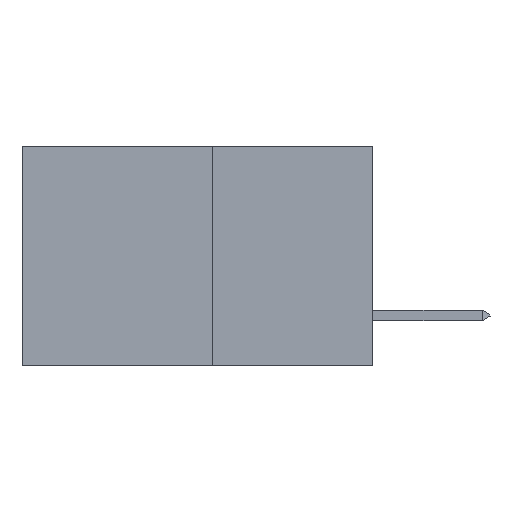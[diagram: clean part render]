
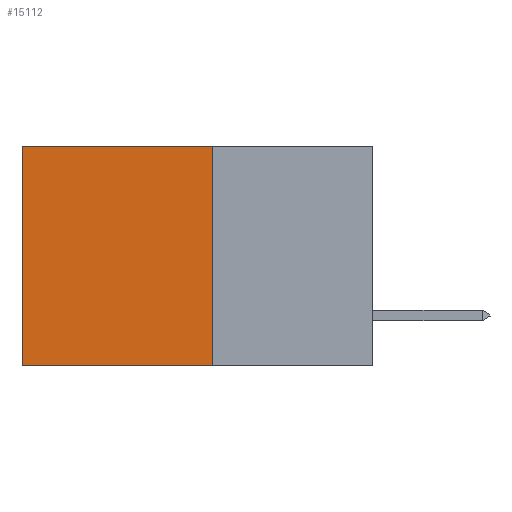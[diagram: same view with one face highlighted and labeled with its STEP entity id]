
A CAD part, left-side view. The second image highlights one B-rep face of the part: STEP entity #15112.
In plain terms, the highlighted planar face has unit normal (-1, 0, 0).
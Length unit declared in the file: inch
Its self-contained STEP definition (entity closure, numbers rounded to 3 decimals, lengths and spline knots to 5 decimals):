
#488 = EDGE_LOOP ( 'NONE', ( #20246, #15571, #25348, #21650 ) ) ;
#1628 = VERTEX_POINT ( 'NONE', #17150 ) ;
#3722 = VECTOR ( 'NONE', #17400, 39.37008 ) ;
#3807 = CARTESIAN_POINT ( 'NONE',  ( 0.277, 0.59, 0. ) ) ;
#5241 = FACE_OUTER_BOUND ( 'NONE', #488, .T. ) ;
#7103 = VERTEX_POINT ( 'NONE', #3807 ) ;
#7363 = VECTOR ( 'NONE', #7800, 39.37008 ) ;
#7687 = CARTESIAN_POINT ( 'NONE',  ( 0.277, 0.59, -0.37 ) ) ;
#7800 = DIRECTION ( 'NONE',  ( 0., 0., -1. ) ) ;
#8806 = DIRECTION ( 'NONE',  ( 0., 1., 0. ) ) ;
#8947 = CARTESIAN_POINT ( 'NONE',  ( 0.277, 0.27, 0. ) ) ;
#9897 = CARTESIAN_POINT ( 'NONE',  ( 0.277, 0.27, -0.37 ) ) ;
#10000 = CARTESIAN_POINT ( 'NONE',  ( 0.277, 0.27, -0.37 ) ) ;
#11214 = EDGE_CURVE ( 'NONE', #18471, #1628, #12854, .T. ) ;
#12854 = LINE ( 'NONE', #15002, #23775 ) ;
#13082 = LINE ( 'NONE', #9897, #7363 ) ;
#13847 = DIRECTION ( 'NONE',  ( 0., 0., -1. ) ) ;
#14249 = LINE ( 'NONE', #7687, #24519 ) ;
#14829 = CARTESIAN_POINT ( 'NONE',  ( 0.277, 0.27, 0. ) ) ;
#15002 = CARTESIAN_POINT ( 'NONE',  ( 0.277, 0.27, -0.37 ) ) ;
#15082 = LINE ( 'NONE', #8947, #3722 ) ;
#15112 = ADVANCED_FACE ( 'NONE', ( #5241 ), #22031, .F. ) ;
#15571 = ORIENTED_EDGE ( 'NONE', *, *, #11214, .F. ) ;
#16810 = AXIS2_PLACEMENT_3D ( 'NONE', #24074, #26175, #13847 ) ;
#17150 = CARTESIAN_POINT ( 'NONE',  ( 0.277, 0.59, -0.37 ) ) ;
#17400 = DIRECTION ( 'NONE',  ( 0., 1., 0. ) ) ;
#18288 = EDGE_CURVE ( 'NONE', #19373, #7103, #15082, .T. ) ;
#18471 = VERTEX_POINT ( 'NONE', #10000 ) ;
#19373 = VERTEX_POINT ( 'NONE', #14829 ) ;
#20246 = ORIENTED_EDGE ( 'NONE', *, *, #24473, .T. ) ;
#21650 = ORIENTED_EDGE ( 'NONE', *, *, #18288, .T. ) ;
#22031 = PLANE ( 'NONE',  #16810 ) ;
#22399 = EDGE_CURVE ( 'NONE', #19373, #18471, #13082, .T. ) ;
#23775 = VECTOR ( 'NONE', #8806, 39.37008 ) ;
#24074 = CARTESIAN_POINT ( 'NONE',  ( 0.277, 0.27, -0.37 ) ) ;
#24354 = DIRECTION ( 'NONE',  ( 0., 0., -1. ) ) ;
#24473 = EDGE_CURVE ( 'NONE', #7103, #1628, #14249, .T. ) ;
#24519 = VECTOR ( 'NONE', #24354, 39.37008 ) ;
#25348 = ORIENTED_EDGE ( 'NONE', *, *, #22399, .F. ) ;
#26175 = DIRECTION ( 'NONE',  ( 1., 0., 0. ) ) ;
